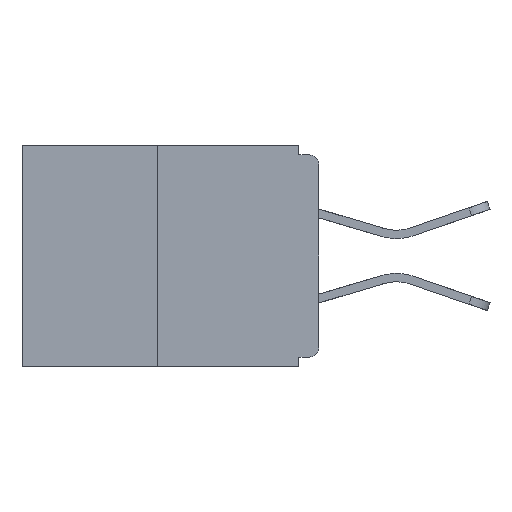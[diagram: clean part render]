
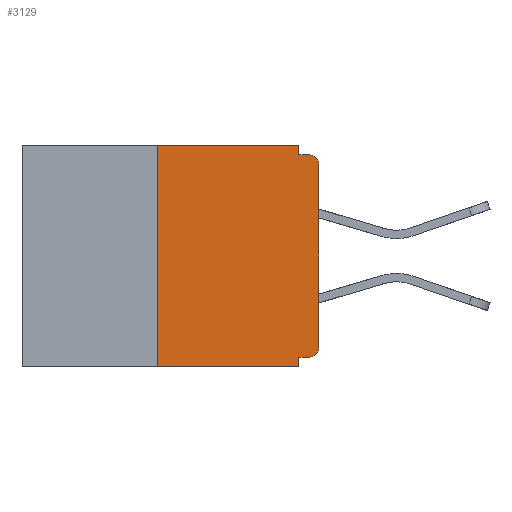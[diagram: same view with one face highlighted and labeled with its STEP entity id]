
A CAD part, left-side view. The second image highlights one B-rep face of the part: STEP entity #3129.
In plain terms, the highlighted planar face has unit normal (-1, 0, 0).
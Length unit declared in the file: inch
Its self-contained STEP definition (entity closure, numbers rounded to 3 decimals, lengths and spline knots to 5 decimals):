
#34 = DIRECTION ( 'NONE',  ( 0., 0., 1. ) ) ;
#571 = LINE ( 'NONE', #8638, #13459 ) ;
#714 = ORIENTED_EDGE ( 'NONE', *, *, #5836, .F. ) ;
#771 = VERTEX_POINT ( 'NONE', #19248 ) ;
#1161 = EDGE_CURVE ( 'NONE', #8558, #5484, #4438, .T. ) ;
#1229 = VERTEX_POINT ( 'NONE', #16061 ) ;
#1762 = ORIENTED_EDGE ( 'NONE', *, *, #5027, .T. ) ;
#2341 = LINE ( 'NONE', #2888, #3299 ) ;
#2582 = CARTESIAN_POINT ( 'NONE',  ( 0., 0.25, 0. ) ) ;
#2888 = CARTESIAN_POINT ( 'NONE',  ( 0., 0., 0. ) ) ;
#2913 = ORIENTED_EDGE ( 'NONE', *, *, #1161, .F. ) ;
#2955 = EDGE_CURVE ( 'NONE', #17237, #5484, #8136, .T. ) ;
#3129 = ADVANCED_FACE ( 'NONE', ( #4591 ), #8459, .F. ) ;
#3299 = VECTOR ( 'NONE', #34, 39.37008 ) ;
#3831 = VECTOR ( 'NONE', #15003, 39.37008 ) ;
#3933 = DIRECTION ( 'NONE',  ( 1., 0., 0. ) ) ;
#4438 = LINE ( 'NONE', #15550, #16663 ) ;
#4585 = ORIENTED_EDGE ( 'NONE', *, *, #9349, .F. ) ;
#4591 = FACE_OUTER_BOUND ( 'NONE', #14095, .T. ) ;
#5027 = EDGE_CURVE ( 'NONE', #5497, #5116, #8276, .T. ) ;
#5116 = VERTEX_POINT ( 'NONE', #6334 ) ;
#5124 = DIRECTION ( 'NONE',  ( 0., 0., -1. ) ) ;
#5302 = VECTOR ( 'NONE', #11679, 39.37008 ) ;
#5476 = LINE ( 'NONE', #9095, #3831 ) ;
#5484 = VERTEX_POINT ( 'NONE', #9990 ) ;
#5497 = VERTEX_POINT ( 'NONE', #18939 ) ;
#5639 = CARTESIAN_POINT ( 'NONE',  ( 0., 0.46, 0. ) ) ;
#5748 = ORIENTED_EDGE ( 'NONE', *, *, #10504, .F. ) ;
#5836 = EDGE_CURVE ( 'NONE', #9187, #9643, #8489, .T. ) ;
#5917 = ORIENTED_EDGE ( 'NONE', *, *, #16531, .F. ) ;
#6334 = CARTESIAN_POINT ( 'NONE',  ( 0., 0., -0.313 ) ) ;
#6433 = EDGE_CURVE ( 'NONE', #5116, #17237, #2341, .T. ) ;
#6503 = VERTEX_POINT ( 'NONE', #7680 ) ;
#6520 = CARTESIAN_POINT ( 'NONE',  ( 0., 0., -0.03 ) ) ;
#6567 = DIRECTION ( 'NONE',  ( 0., -1., 0. ) ) ;
#6986 = LINE ( 'NONE', #2582, #11684 ) ;
#7265 = CARTESIAN_POINT ( 'NONE',  ( 0., 0.031, -0.343 ) ) ;
#7471 = VECTOR ( 'NONE', #13847, 39.37008 ) ;
#7570 = VECTOR ( 'NONE', #10521, 39.37008 ) ;
#7680 = CARTESIAN_POINT ( 'NONE',  ( 0., 0.25, -0.343 ) ) ;
#8136 = CIRCLE ( 'NONE', #17232, 0.015 ) ;
#8276 = CIRCLE ( 'NONE', #9717, 0.015 ) ;
#8338 = DIRECTION ( 'NONE',  ( -1., 0., 0. ) ) ;
#8459 = PLANE ( 'NONE',  #11087 ) ;
#8489 = LINE ( 'NONE', #14917, #7570 ) ;
#8558 = VERTEX_POINT ( 'NONE', #11134 ) ;
#8638 = CARTESIAN_POINT ( 'NONE',  ( 0., 0.031, 0. ) ) ;
#9046 = LINE ( 'NONE', #17785, #5302 ) ;
#9095 = CARTESIAN_POINT ( 'NONE',  ( 0., 0.46, 0. ) ) ;
#9187 = VERTEX_POINT ( 'NONE', #12932 ) ;
#9349 = EDGE_CURVE ( 'NONE', #5497, #9187, #9046, .T. ) ;
#9394 = DIRECTION ( 'NONE',  ( 0., 0., -1. ) ) ;
#9530 = CARTESIAN_POINT ( 'NONE',  ( 0., 0.015, -0.313 ) ) ;
#9643 = VERTEX_POINT ( 'NONE', #7265 ) ;
#9717 = AXIS2_PLACEMENT_3D ( 'NONE', #9530, #11046, #9394 ) ;
#9990 = CARTESIAN_POINT ( 'NONE',  ( 0., 0.015, -0.015 ) ) ;
#10386 = EDGE_CURVE ( 'NONE', #771, #8558, #571, .T. ) ;
#10445 = ORIENTED_EDGE ( 'NONE', *, *, #15670, .T. ) ;
#10504 = EDGE_CURVE ( 'NONE', #1229, #771, #5476, .T. ) ;
#10521 = DIRECTION ( 'NONE',  ( 0., 0., -1. ) ) ;
#11046 = DIRECTION ( 'NONE',  ( -1., 0., 0. ) ) ;
#11087 = AXIS2_PLACEMENT_3D ( 'NONE', #5639, #3933, #16211 ) ;
#11134 = CARTESIAN_POINT ( 'NONE',  ( 0., 0.031, -0.015 ) ) ;
#11278 = ORIENTED_EDGE ( 'NONE', *, *, #10386, .F. ) ;
#11670 = DIRECTION ( 'NONE',  ( 0., 0., -1. ) ) ;
#11679 = DIRECTION ( 'NONE',  ( 0., 1., 0. ) ) ;
#11684 = VECTOR ( 'NONE', #18245, 39.37008 ) ;
#12811 = CARTESIAN_POINT ( 'NONE',  ( 0., 0.015, -0.03 ) ) ;
#12932 = CARTESIAN_POINT ( 'NONE',  ( 0., 0.031, -0.328 ) ) ;
#13459 = VECTOR ( 'NONE', #11670, 39.37008 ) ;
#13847 = DIRECTION ( 'NONE',  ( 0., -1., 0. ) ) ;
#14095 = EDGE_LOOP ( 'NONE', ( #5748, #5917, #10445, #714, #4585, #1762, #14808, #16772, #2913, #11278 ) ) ;
#14103 = CARTESIAN_POINT ( 'NONE',  ( 0., 0.46, -0.343 ) ) ;
#14808 = ORIENTED_EDGE ( 'NONE', *, *, #6433, .T. ) ;
#14917 = CARTESIAN_POINT ( 'NONE',  ( 0., 0.031, -0.343 ) ) ;
#14973 = LINE ( 'NONE', #14103, #7471 ) ;
#15003 = DIRECTION ( 'NONE',  ( 0., -1., 0. ) ) ;
#15550 = CARTESIAN_POINT ( 'NONE',  ( 0., 0., -0.015 ) ) ;
#15670 = EDGE_CURVE ( 'NONE', #6503, #9643, #14973, .T. ) ;
#16061 = CARTESIAN_POINT ( 'NONE',  ( 0., 0.25, 0. ) ) ;
#16211 = DIRECTION ( 'NONE',  ( 0., 0., -1. ) ) ;
#16531 = EDGE_CURVE ( 'NONE', #6503, #1229, #6986, .T. ) ;
#16663 = VECTOR ( 'NONE', #6567, 39.37008 ) ;
#16772 = ORIENTED_EDGE ( 'NONE', *, *, #2955, .T. ) ;
#17232 = AXIS2_PLACEMENT_3D ( 'NONE', #12811, #8338, #5124 ) ;
#17237 = VERTEX_POINT ( 'NONE', #6520 ) ;
#17785 = CARTESIAN_POINT ( 'NONE',  ( 0., 0., -0.328 ) ) ;
#18245 = DIRECTION ( 'NONE',  ( 0., 0., 1. ) ) ;
#18939 = CARTESIAN_POINT ( 'NONE',  ( 0., 0.015, -0.328 ) ) ;
#19248 = CARTESIAN_POINT ( 'NONE',  ( 0., 0.031, 0. ) ) ;
